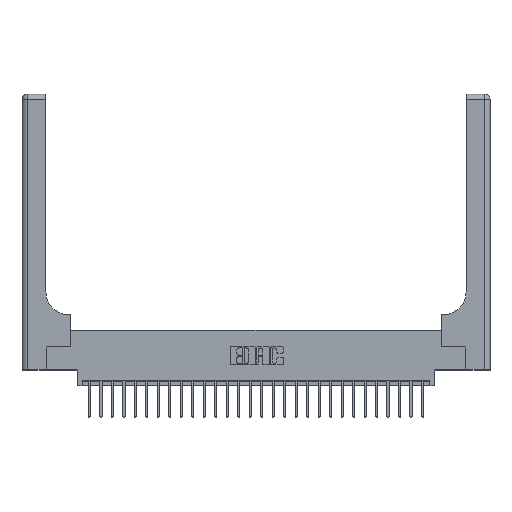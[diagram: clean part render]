
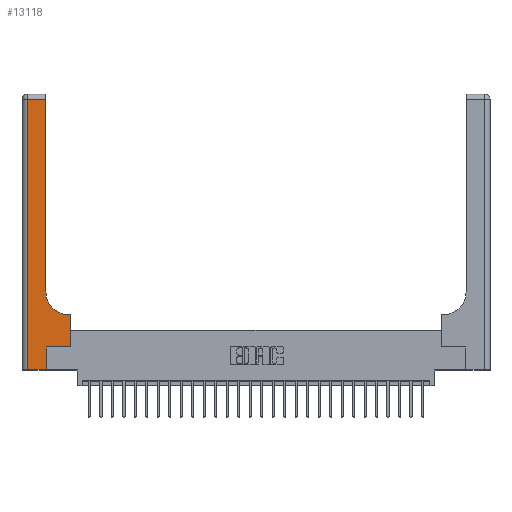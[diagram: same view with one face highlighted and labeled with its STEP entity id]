
A CAD part, top view. The second image highlights one B-rep face of the part: STEP entity #13118.
In plain terms, the highlighted planar face has unit normal (0, 0, 1).
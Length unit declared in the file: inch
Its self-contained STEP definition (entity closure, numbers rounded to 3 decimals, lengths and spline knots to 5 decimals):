
#9 = LINE ( 'NONE', #9919, #16528 ) ;
#45 = LINE ( 'NONE', #7265, #20682 ) ;
#456 = CARTESIAN_POINT ( 'NONE',  ( 0.06, 0., 0.37 ) ) ;
#784 = EDGE_CURVE ( 'NONE', #5274, #6730, #9, .T. ) ;
#1345 = CARTESIAN_POINT ( 'NONE',  ( 0.26, 0.6, 0.37 ) ) ;
#1368 = CARTESIAN_POINT ( 'NONE',  ( 0.528, 0.25, 0.37 ) ) ;
#1808 = VERTEX_POINT ( 'NONE', #17351 ) ;
#2705 = CARTESIAN_POINT ( 'NONE',  ( 0.26, 2.94, 0.37 ) ) ;
#3325 = EDGE_CURVE ( 'NONE', #20533, #8596, #7569, .T. ) ;
#3397 = DIRECTION ( 'NONE',  ( 0., 1., 0. ) ) ;
#3430 = DIRECTION ( 'NONE',  ( -1., 0., 0. ) ) ;
#3494 = CARTESIAN_POINT ( 'NONE',  ( 0., 2.94, 0.37 ) ) ;
#3598 = DIRECTION ( 'NONE',  ( 0., 0., -1. ) ) ;
#3861 = VECTOR ( 'NONE', #3430, 39.37008 ) ;
#4267 = CIRCLE ( 'NONE', #13641, 0.25 ) ;
#4418 = EDGE_CURVE ( 'NONE', #6730, #14224, #45, .T. ) ;
#5186 = EDGE_CURVE ( 'NONE', #1808, #20533, #10428, .T. ) ;
#5274 = VERTEX_POINT ( 'NONE', #20172 ) ;
#5605 = DIRECTION ( 'NONE',  ( -1., 0., 0. ) ) ;
#6730 = VERTEX_POINT ( 'NONE', #20098 ) ;
#6793 = FACE_OUTER_BOUND ( 'NONE', #10833, .T. ) ;
#6995 = CARTESIAN_POINT ( 'NONE',  ( 0.51, 0.85, 0.37 ) ) ;
#7265 = CARTESIAN_POINT ( 'NONE',  ( 0.265, 0.25, 0.37 ) ) ;
#7569 = LINE ( 'NONE', #3494, #22651 ) ;
#8596 = VERTEX_POINT ( 'NONE', #22842 ) ;
#8602 = CARTESIAN_POINT ( 'NONE',  ( 0.528, 0.25, 0.37 ) ) ;
#8903 = CARTESIAN_POINT ( 'NONE',  ( 0.51, 0.6, 0.37 ) ) ;
#9071 = DIRECTION ( 'NONE',  ( 1., 0., 0. ) ) ;
#9592 = CARTESIAN_POINT ( 'NONE',  ( 0., 0., 0.37 ) ) ;
#9919 = CARTESIAN_POINT ( 'NONE',  ( 0.265, 0., 0.37 ) ) ;
#10428 = LINE ( 'NONE', #23903, #15257 ) ;
#10809 = ORIENTED_EDGE ( 'NONE', *, *, #25378, .T. ) ;
#10833 = EDGE_LOOP ( 'NONE', ( #15159, #16699, #16568, #12999, #18718, #13457, #21904, #10809, #16932 ) ) ;
#11682 = EDGE_CURVE ( 'NONE', #8596, #15617, #18493, .T. ) ;
#12850 = DIRECTION ( 'NONE',  ( 0., 1., 0. ) ) ;
#12999 = ORIENTED_EDGE ( 'NONE', *, *, #13070, .T. ) ;
#13070 = EDGE_CURVE ( 'NONE', #15617, #5274, #24439, .T. ) ;
#13118 = ADVANCED_FACE ( 'NONE', ( #6793 ), #20022, .F. ) ;
#13455 = EDGE_CURVE ( 'NONE', #14224, #19845, #21562, .T. ) ;
#13457 = ORIENTED_EDGE ( 'NONE', *, *, #4418, .T. ) ;
#13473 = AXIS2_PLACEMENT_3D ( 'NONE', #16017, #3598, #18070 ) ;
#13641 = AXIS2_PLACEMENT_3D ( 'NONE', #6995, #21370, #9071 ) ;
#14224 = VERTEX_POINT ( 'NONE', #1368 ) ;
#14495 = CARTESIAN_POINT ( 'NONE',  ( 0.06, 3., 0.37 ) ) ;
#15159 = ORIENTED_EDGE ( 'NONE', *, *, #5186, .T. ) ;
#15257 = VECTOR ( 'NONE', #3397, 39.37008 ) ;
#15617 = VERTEX_POINT ( 'NONE', #456 ) ;
#16017 = CARTESIAN_POINT ( 'NONE',  ( 0., 3., 0.37 ) ) ;
#16173 = VECTOR ( 'NONE', #12850, 39.37008 ) ;
#16528 = VECTOR ( 'NONE', #22212, 39.37008 ) ;
#16568 = ORIENTED_EDGE ( 'NONE', *, *, #11682, .T. ) ;
#16665 = DIRECTION ( 'NONE',  ( 0., -1., 0. ) ) ;
#16699 = ORIENTED_EDGE ( 'NONE', *, *, #3325, .T. ) ;
#16932 = ORIENTED_EDGE ( 'NONE', *, *, #23505, .T. ) ;
#17204 = VECTOR ( 'NONE', #16665, 39.37008 ) ;
#17351 = CARTESIAN_POINT ( 'NONE',  ( 0.26, 0.85, 0.37 ) ) ;
#18070 = DIRECTION ( 'NONE',  ( -1., 0., 0. ) ) ;
#18493 = LINE ( 'NONE', #14495, #17204 ) ;
#18547 = VERTEX_POINT ( 'NONE', #8903 ) ;
#18718 = ORIENTED_EDGE ( 'NONE', *, *, #784, .T. ) ;
#19052 = VECTOR ( 'NONE', #25926, 39.37008 ) ;
#19845 = VERTEX_POINT ( 'NONE', #23253 ) ;
#20022 = PLANE ( 'NONE',  #13473 ) ;
#20098 = CARTESIAN_POINT ( 'NONE',  ( 0.265, 0.25, 0.37 ) ) ;
#20172 = CARTESIAN_POINT ( 'NONE',  ( 0.265, 0., 0.37 ) ) ;
#20533 = VERTEX_POINT ( 'NONE', #2705 ) ;
#20682 = VECTOR ( 'NONE', #23663, 39.37008 ) ;
#21370 = DIRECTION ( 'NONE',  ( 0., 0., -1. ) ) ;
#21562 = LINE ( 'NONE', #8602, #16173 ) ;
#21904 = ORIENTED_EDGE ( 'NONE', *, *, #13455, .T. ) ;
#22212 = DIRECTION ( 'NONE',  ( 0., 1., 0. ) ) ;
#22651 = VECTOR ( 'NONE', #5605, 39.37008 ) ;
#22842 = CARTESIAN_POINT ( 'NONE',  ( 0.06, 2.94, 0.37 ) ) ;
#23253 = CARTESIAN_POINT ( 'NONE',  ( 0.528, 0.6, 0.37 ) ) ;
#23505 = EDGE_CURVE ( 'NONE', #18547, #1808, #4267, .T. ) ;
#23663 = DIRECTION ( 'NONE',  ( 1., 0., 0. ) ) ;
#23903 = CARTESIAN_POINT ( 'NONE',  ( 0.26, 3., 0.37 ) ) ;
#24439 = LINE ( 'NONE', #9592, #19052 ) ;
#25378 = EDGE_CURVE ( 'NONE', #19845, #18547, #25671, .T. ) ;
#25671 = LINE ( 'NONE', #1345, #3861 ) ;
#25926 = DIRECTION ( 'NONE',  ( 1., 0., 0. ) ) ;
